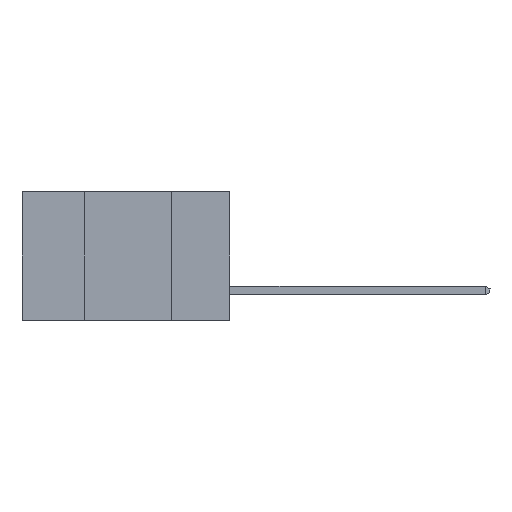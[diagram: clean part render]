
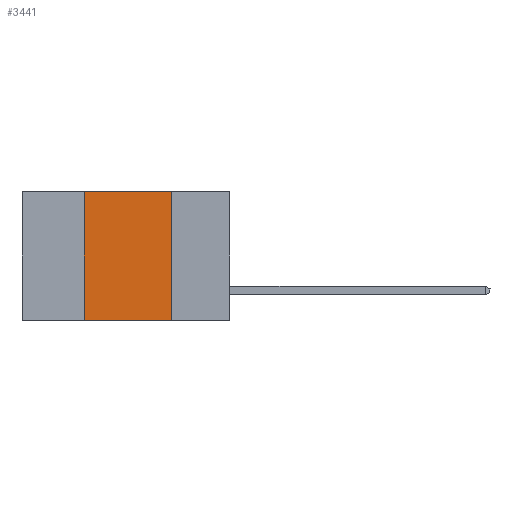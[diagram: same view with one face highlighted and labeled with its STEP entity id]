
A CAD part, left-side view. The second image highlights one B-rep face of the part: STEP entity #3441.
In plain terms, the highlighted planar face has unit normal (-1, 0, 0).
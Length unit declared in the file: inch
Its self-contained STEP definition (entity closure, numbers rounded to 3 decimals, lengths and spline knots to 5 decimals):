
#64 = VECTOR ( 'NONE', #793, 39.37008 ) ;
#235 = AXIS2_PLACEMENT_3D ( 'NONE', #7772, #1500, #15185 ) ;
#241 = VERTEX_POINT ( 'NONE', #4537 ) ;
#339 = EDGE_LOOP ( 'NONE', ( #5347, #11556, #15474, #3905 ) ) ;
#512 = EDGE_CURVE ( 'NONE', #4848, #241, #7631, .T. ) ;
#793 = DIRECTION ( 'NONE',  ( 0., 0., 1. ) ) ;
#1500 = DIRECTION ( 'NONE',  ( 1., 0., 0. ) ) ;
#3005 = LINE ( 'NONE', #7043, #6240 ) ;
#3303 = LINE ( 'NONE', #8433, #9319 ) ;
#3441 = ADVANCED_FACE ( 'NONE', ( #10442 ), #10278, .F. ) ;
#3614 = CARTESIAN_POINT ( 'NONE',  ( 0., 0.42, -0.37 ) ) ;
#3729 = EDGE_CURVE ( 'NONE', #5243, #7744, #3303, .T. ) ;
#3853 = DIRECTION ( 'NONE',  ( 0., -1., 0. ) ) ;
#3905 = ORIENTED_EDGE ( 'NONE', *, *, #3729, .T. ) ;
#4537 = CARTESIAN_POINT ( 'NONE',  ( 0., 0.17, 0. ) ) ;
#4848 = VERTEX_POINT ( 'NONE', #9609 ) ;
#4894 = LINE ( 'NONE', #3614, #64 ) ;
#5115 = VECTOR ( 'NONE', #3853, 39.37008 ) ;
#5243 = VERTEX_POINT ( 'NONE', #14252 ) ;
#5347 = ORIENTED_EDGE ( 'NONE', *, *, #15566, .F. ) ;
#6240 = VECTOR ( 'NONE', #8122, 39.37008 ) ;
#7043 = CARTESIAN_POINT ( 'NONE',  ( 0., 0.17, -0.37 ) ) ;
#7631 = LINE ( 'NONE', #12885, #5115 ) ;
#7744 = VERTEX_POINT ( 'NONE', #10204 ) ;
#7772 = CARTESIAN_POINT ( 'NONE',  ( 0., 0.6, 0. ) ) ;
#8122 = DIRECTION ( 'NONE',  ( 0., 0., -1. ) ) ;
#8433 = CARTESIAN_POINT ( 'NONE',  ( 0., 0.6, -0.37 ) ) ;
#9319 = VECTOR ( 'NONE', #12341, 39.37008 ) ;
#9609 = CARTESIAN_POINT ( 'NONE',  ( 0., 0.42, 0. ) ) ;
#10204 = CARTESIAN_POINT ( 'NONE',  ( 0., 0.17, -0.37 ) ) ;
#10278 = PLANE ( 'NONE',  #235 ) ;
#10442 = FACE_OUTER_BOUND ( 'NONE', #339, .T. ) ;
#11556 = ORIENTED_EDGE ( 'NONE', *, *, #512, .F. ) ;
#12341 = DIRECTION ( 'NONE',  ( 0., -1., 0. ) ) ;
#12872 = EDGE_CURVE ( 'NONE', #5243, #4848, #4894, .T. ) ;
#12885 = CARTESIAN_POINT ( 'NONE',  ( 0., 0.6, 0. ) ) ;
#14252 = CARTESIAN_POINT ( 'NONE',  ( 0., 0.42, -0.37 ) ) ;
#15185 = DIRECTION ( 'NONE',  ( 0., 0., -1. ) ) ;
#15474 = ORIENTED_EDGE ( 'NONE', *, *, #12872, .F. ) ;
#15566 = EDGE_CURVE ( 'NONE', #241, #7744, #3005, .T. ) ;
